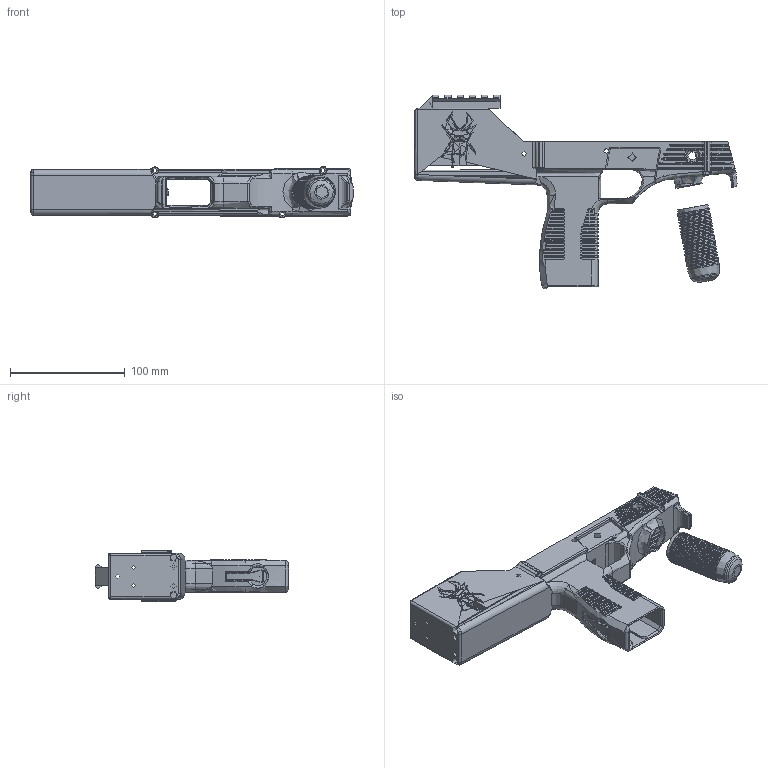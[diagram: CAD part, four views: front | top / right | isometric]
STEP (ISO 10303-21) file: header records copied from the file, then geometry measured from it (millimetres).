
FILE_DESCRIPTION(/* description */ (''),/* implementation_level */ '2;1');
FILE_NAME(/* name */ 'Scarab DMB Remix.step',/* time_stamp */ '2022-05-05T01:57:43-04:00',/* author */ (''),/* organization */ (''),/* preprocessor_version */ 'ST-DEVELOPER v18.1',/* originating_system */ 'Autodesk Translation Framework v10.14.0.1471',/* authorisation */ '');
FILE_SCHEMA (('AUTOMOTIVE_DESIGN { 1 0 10303 214 3 1 1 }'));
Products named in the file (1): Scarab
Bounding box: 280.32 x 168.37 x 44.61 mm (x, y, z)
Volume: 1148.7 mm3; surface area: 119818.2 mm2
Topology: 7 solids, 8 shells, 2403 faces, 5961 edges, 3627 vertices
Faces by surface type: cylinder 724, plane 715, bspline 574, torus 383, cone 5, sphere 2
Full cylindrical faces by diameter (mm): 2.2 x3, 3.073 x4, 3.4 x1, 3.5 x2, 4.089 x2, 4.7 x6, 4.75 x1, 4.757 x1, 5.5 x1, 5.588 x1, 6.096 x1, 6.2 x1, 6.35 x1, 6.604 x1, 7.417 x1, 7.62 x1, 7.95 x1, 8.255 x2, 11.2 x1, 26.924 x20, 28.475 x20
Entity records: 218623 total; most frequent: CARTESIAN_POINT 164323, ORIENTED_EDGE 11864, DIRECTION 10571, EDGE_CURVE 5932, AXIS2_PLACEMENT_3D 4125, VERTEX_POINT 3627, EDGE_LOOP 2541, FACE_OUTER_BOUND 2403
